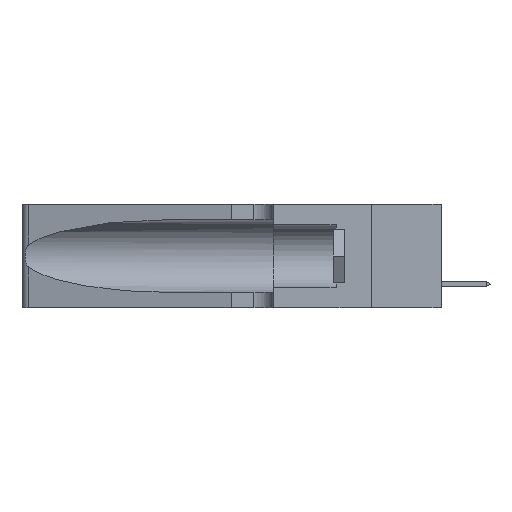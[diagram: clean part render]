
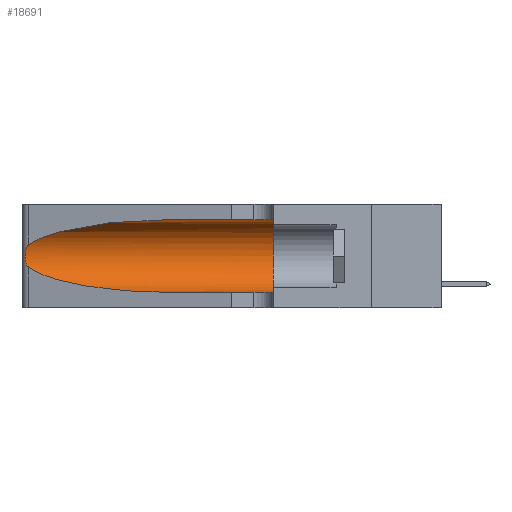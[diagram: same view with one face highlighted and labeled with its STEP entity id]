
A CAD part, left-side view. The second image highlights one B-rep face of the part: STEP entity #18691.
In plain terms, the highlighted cylindrical face has radius 3.308 mm (diameter 6.617 mm), a partial arc.
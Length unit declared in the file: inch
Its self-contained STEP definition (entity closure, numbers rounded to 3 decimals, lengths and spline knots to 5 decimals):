
#405 = DIRECTION ( 'NONE',  ( 0., 1., 0. ) ) ;
#1208 = CARTESIAN_POINT ( 'NONE',  ( 0.25639, 1.23184, 0.21858 ) ) ;
#1248 = CARTESIAN_POINT ( 'NONE',  ( 0.1305, 1.61858, 0.05475 ) ) ;
#1515 = CARTESIAN_POINT ( 'NONE',  ( 0.25487, 1.22718, 0.14631 ) ) ;
#1564 = CARTESIAN_POINT ( 'NONE',  ( 0.18966, 0.96281, 0.05475 ) ) ;
#2179 = ORIENTED_EDGE ( 'NONE', *, *, #8267, .F. ) ;
#2716 = CARTESIAN_POINT ( 'NONE',  ( 0.1305, 1.61858, 0.31525 ) ) ;
#2823 = VECTOR ( 'NONE', #22687, 39.37008 ) ;
#3098 = CARTESIAN_POINT ( 'NONE',  ( 0.1305, 0.72297, 0.05475 ) ) ;
#3562 = CARTESIAN_POINT ( 'NONE',  ( 0.25639, 1.23186, 0.15144 ) ) ;
#4819 = CARTESIAN_POINT ( 'NONE',  ( 0.25854, 1.2359, 0.20912 ) ) ;
#5359 = LINE ( 'NONE', #2716, #2823 ) ;
#6412 = ORIENTED_EDGE ( 'NONE', *, *, #7613, .F. ) ;
#6773 = EDGE_CURVE ( 'NONE', #7826, #15466, #7686, .T. ) ;
#6941 = DIRECTION ( 'NONE',  ( 0., -1., 0. ) ) ;
#7168 = CARTESIAN_POINT ( 'NONE',  ( 0.25789, 1.23486, 0.15765 ) ) ;
#7356 = CARTESIAN_POINT ( 'NONE',  ( 0.2373, 1.15595, 0.08982 ) ) ;
#7613 = EDGE_CURVE ( 'NONE', #7826, #9397, #5359, .T. ) ;
#7631 = CARTESIAN_POINT ( 'NONE',  ( 0.1305, 0.35, 0.185 ) ) ;
#7686 =( BOUNDED_CURVE ( )  B_SPLINE_CURVE ( 3, ( #9696, #9531, #22278, #11494 ),
 .UNSPECIFIED., .F., .T. ) 
 B_SPLINE_CURVE_WITH_KNOTS ( ( 4, 4 ),
 ( 1.5708, 2.84003 ),
 .UNSPECIFIED. ) 
 CURVE ( )  GEOMETRIC_REPRESENTATION_ITEM ( )  RATIONAL_B_SPLINE_CURVE ( ( 1., 0.87, 0.87, 1. ) ) 
 REPRESENTATION_ITEM ( '' )  );
#7714 = DIRECTION ( 'NONE',  ( 0., 0., 1. ) ) ;
#7826 = VERTEX_POINT ( 'NONE', #10017 ) ;
#8039 = CARTESIAN_POINT ( 'NONE',  ( 0.1305, 0.35, 0.05475 ) ) ;
#8267 = EDGE_CURVE ( 'NONE', #9397, #15774, #19228, .T. ) ;
#8397 = CARTESIAN_POINT ( 'NONE',  ( 0.25487, 1.22718, 0.22369 ) ) ;
#8721 = AXIS2_PLACEMENT_3D ( 'NONE', #18373, #12925, #20175 ) ;
#8755 = CARTESIAN_POINT ( 'NONE',  ( 0.1305, 0.35, 0.31525 ) ) ;
#9397 = VERTEX_POINT ( 'NONE', #8755 ) ;
#9531 = CARTESIAN_POINT ( 'NONE',  ( 0.18966, 0.96281, 0.31525 ) ) ;
#9696 = CARTESIAN_POINT ( 'NONE',  ( 0.1305, 0.72297, 0.31525 ) ) ;
#10017 = CARTESIAN_POINT ( 'NONE',  ( 0.1305, 0.72297, 0.31525 ) ) ;
#10413 = CARTESIAN_POINT ( 'NONE',  ( 0.25487, 1.22718, 0.22369 ) ) ;
#10709 = CARTESIAN_POINT ( 'NONE',  ( 0.26075, 1.23896, 0.19203 ) ) ;
#10844 = ORIENTED_EDGE ( 'NONE', *, *, #11373, .T. ) ;
#11373 = EDGE_CURVE ( 'NONE', #13068, #15774, #17651, .T. ) ;
#11391 = FACE_OUTER_BOUND ( 'NONE', #21147, .T. ) ;
#11494 = CARTESIAN_POINT ( 'NONE',  ( 0.25487, 1.22718, 0.22369 ) ) ;
#12246 = CARTESIAN_POINT ( 'NONE',  ( 0.25555, 1.22993, 0.14849 ) ) ;
#12925 = DIRECTION ( 'NONE',  ( 0., -1., 0. ) ) ;
#13068 = VERTEX_POINT ( 'NONE', #3098 ) ;
#13829 = CARTESIAN_POINT ( 'NONE',  ( 0.25787, 1.23484, 0.2124 ) ) ;
#14279 = CARTESIAN_POINT ( 'NONE',  ( 0.1305, 0.72297, 0.05475 ) ) ;
#14400 = CARTESIAN_POINT ( 'NONE',  ( 0.26075, 1.23896, 0.178 ) ) ;
#14519 = CARTESIAN_POINT ( 'NONE',  ( 0.25487, 1.22718, 0.14631 ) ) ;
#15466 = VERTEX_POINT ( 'NONE', #10413 ) ;
#15774 = VERTEX_POINT ( 'NONE', #8039 ) ;
#16145 = CARTESIAN_POINT ( 'NONE',  ( 0.26017, 1.23833, 0.17102 ) ) ;
#17471 = CARTESIAN_POINT ( 'NONE',  ( 0.26018, 1.23835, 0.19895 ) ) ;
#17584 = ORIENTED_EDGE ( 'NONE', *, *, #17604, .T. ) ;
#17604 = EDGE_CURVE ( 'NONE', #20668, #13068, #18516, .T. ) ;
#17651 = LINE ( 'NONE', #1248, #18492 ) ;
#17786 = CARTESIAN_POINT ( 'NONE',  ( 0.25856, 1.23593, 0.16098 ) ) ;
#18373 = CARTESIAN_POINT ( 'NONE',  ( 0.1305, 1.61858, 0.185 ) ) ;
#18492 = VECTOR ( 'NONE', #6941, 39.37008 ) ;
#18516 =( BOUNDED_CURVE ( )  B_SPLINE_CURVE ( 3, ( #14519, #7356, #1564, #14279 ),
 .UNSPECIFIED., .F., .F. ) 
 B_SPLINE_CURVE_WITH_KNOTS ( ( 4, 4 ),
 ( 3.44316, 4.71239 ),
 .UNSPECIFIED. ) 
 CURVE ( )  GEOMETRIC_REPRESENTATION_ITEM ( )  RATIONAL_B_SPLINE_CURVE ( ( 1., 0.87, 0.87, 1. ) ) 
 REPRESENTATION_ITEM ( '' )  );
#18691 = ADVANCED_FACE ( 'NONE', ( #11391 ), #20397, .F. ) ;
#18950 = ORIENTED_EDGE ( 'NONE', *, *, #6773, .T. ) ;
#19228 = CIRCLE ( 'NONE', #20599, 0.13025 ) ;
#19618 = CARTESIAN_POINT ( 'NONE',  ( 0.25487, 1.22718, 0.14631 ) ) ;
#20175 = DIRECTION ( 'NONE',  ( 0., 0., -1. ) ) ;
#20219 = EDGE_CURVE ( 'NONE', #15466, #20668, #20626, .T. ) ;
#20397 = CYLINDRICAL_SURFACE ( 'NONE', #8721, 0.13025 ) ;
#20599 = AXIS2_PLACEMENT_3D ( 'NONE', #7631, #405, #7714 ) ;
#20626 = B_SPLINE_CURVE_WITH_KNOTS ( 'NONE', 3,
 ( #8397, #22751, #1208, #13829, #4819, #17471, #10709, #14400, #16145, #17786, #7168, #3562, #12246, #1515 ),
 .UNSPECIFIED., .F., .F.,
 ( 4, 2, 2, 2, 2, 2, 4 ),
 ( 0., 0.00027, 0.00053, 0.00107, 0.0016, 0.00187, 0.00214 ),
 .UNSPECIFIED. ) ;
#20668 = VERTEX_POINT ( 'NONE', #19618 ) ;
#21147 = EDGE_LOOP ( 'NONE', ( #18950, #22365, #17584, #10844, #2179, #6412 ) ) ;
#22278 = CARTESIAN_POINT ( 'NONE',  ( 0.2373, 1.15595, 0.28018 ) ) ;
#22365 = ORIENTED_EDGE ( 'NONE', *, *, #20219, .T. ) ;
#22687 = DIRECTION ( 'NONE',  ( 0., -1., 0. ) ) ;
#22751 = CARTESIAN_POINT ( 'NONE',  ( 0.25555, 1.22994, 0.2215 ) ) ;
